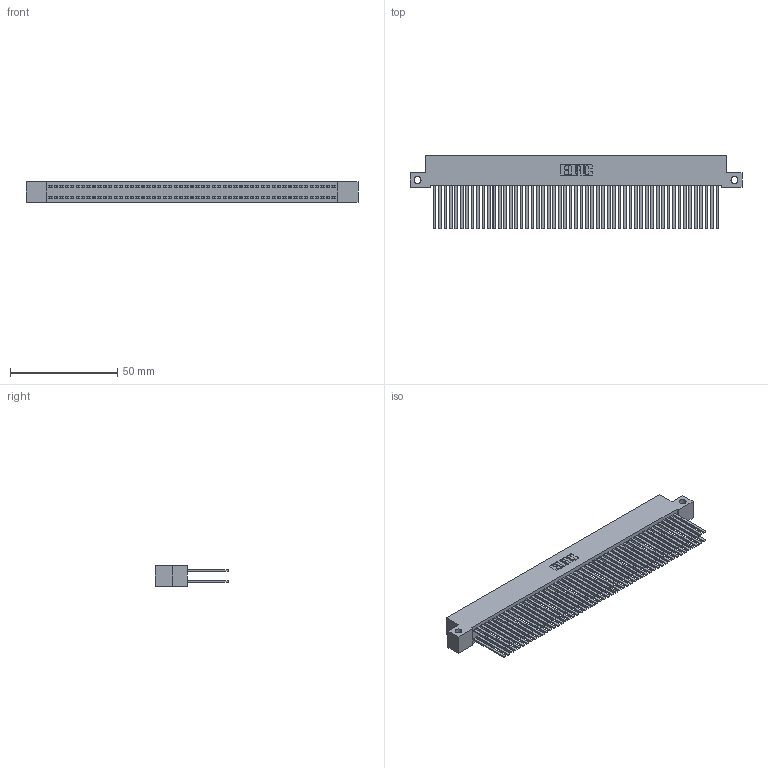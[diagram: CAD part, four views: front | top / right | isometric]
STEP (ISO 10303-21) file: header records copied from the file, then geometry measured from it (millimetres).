
FILE_DESCRIPTION (( 'STEP AP203' ), '1' );
FILE_NAME ('342-106-544-212.STEP', '2018-08-14T07:08:11', ( '' ), ( '' ), 'SwSTEP 2.0', 'SolidWorks 2016', '' );
FILE_SCHEMA (( 'CONFIG_CONTROL_DESIGN' ));
Length unit declared in the file: inch
Products named in the file (3): 342-106-544-212; 342 Part_Side Mount; 345-292-001_345-293-144
Assembly tree (107 placements, depth 2):
  342-106-544-212
    342 Part_Side Mount
    345-292-001_345-293-144  x106
Bounding box: 154.94 x 34.3 x 9.4 mm (x, y, z)
Volume: 15385.4 mm3; surface area: 29269.9 mm2
Topology: 107 solids, 107 shells, 4986 faces, 14821 edges, 9738 vertices
Faces by surface type: plane 3458, cylinder 1528
Entity records: 32361 total; most frequent: CARTESIAN_POINT 5346, ORIENTED_EDGE 5282, DIRECTION 4545, EDGE_CURVE 2641, VECTOR 2517, LINE 2517, VERTEX_POINT 1758, AXIS2_PLACEMENT_3D 1014
